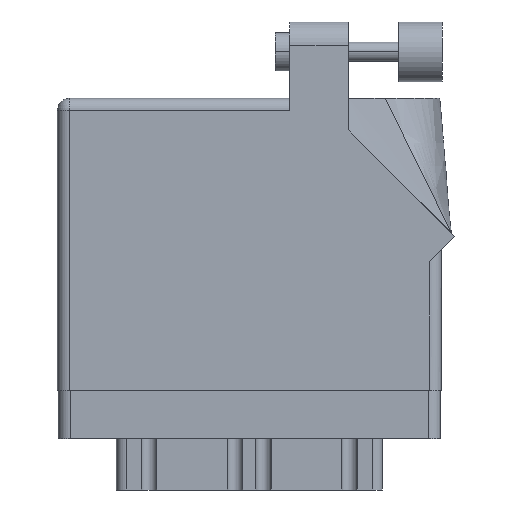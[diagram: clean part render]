
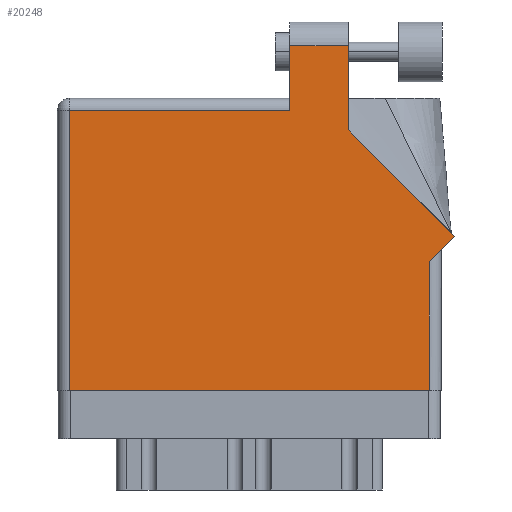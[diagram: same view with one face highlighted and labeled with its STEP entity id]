
A CAD part, front view. The second image highlights one B-rep face of the part: STEP entity #20248.
In plain terms, the highlighted face is planar.
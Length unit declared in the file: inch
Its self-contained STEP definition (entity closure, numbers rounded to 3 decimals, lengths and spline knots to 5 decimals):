
#191 = CARTESIAN_POINT ( 'NONE',  ( 1.948, 0., 0. ) ) ;
#868 = CARTESIAN_POINT ( 'NONE',  ( 2.08071, 0.80771, 0. ) ) ;
#1690 = CARTESIAN_POINT ( 'NONE',  ( 0., 1.53, 0. ) ) ;
#2049 = DIRECTION ( 'NONE',  ( 0., -1., 0. ) ) ;
#2469 = VECTOR ( 'NONE', #13653, 39.37008 ) ;
#2564 = EDGE_CURVE ( 'NONE', #34526, #6730, #16351, .T. ) ;
#2568 = CARTESIAN_POINT ( 'NONE',  ( 1.948, 0.737, 0. ) ) ;
#2931 = CARTESIAN_POINT ( 'NONE',  ( 1.524, 1.36442, 0. ) ) ;
#4004 = LINE ( 'NONE', #868, #5457 ) ;
#4192 = VECTOR ( 'NONE', #5695, 39.37008 ) ;
#4237 = DIRECTION ( 'NONE',  ( 0., 0., -1. ) ) ;
#4546 = ORIENTED_EDGE ( 'NONE', *, *, #4769, .T. ) ;
#4769 = EDGE_CURVE ( 'NONE', #14271, #34526, #4004, .T. ) ;
#4991 = VECTOR ( 'NONE', #36808, 39.37008 ) ;
#5081 = ORIENTED_EDGE ( 'NONE', *, *, #16974, .T. ) ;
#5451 = DIRECTION ( 'NONE',  ( -1., 0., 0. ) ) ;
#5457 = VECTOR ( 'NONE', #15938, 39.37008 ) ;
#5651 = EDGE_CURVE ( 'NONE', #19628, #32296, #12867, .T. ) ;
#5695 = DIRECTION ( 'NONE',  ( 0., 1., 0. ) ) ;
#6150 = EDGE_CURVE ( 'NONE', #12556, #30649, #23180, .T. ) ;
#6730 = VERTEX_POINT ( 'NONE', #27021 ) ;
#9202 = CARTESIAN_POINT ( 'NONE',  ( 2.01, 0.737, 0. ) ) ;
#9507 = DIRECTION ( 'NONE',  ( -1., 0., 0. ) ) ;
#10709 = EDGE_CURVE ( 'NONE', #12248, #14271, #27019, .T. ) ;
#11856 = AXIS2_PLACEMENT_3D ( 'NONE', #1690, #4237, #34006 ) ;
#12248 = VERTEX_POINT ( 'NONE', #29646 ) ;
#12556 = VERTEX_POINT ( 'NONE', #23153 ) ;
#12867 = LINE ( 'NONE', #22465, #2469 ) ;
#12920 = CARTESIAN_POINT ( 'NONE',  ( 0.062, 0., 0. ) ) ;
#12975 = ORIENTED_EDGE ( 'NONE', *, *, #19681, .T. ) ;
#13653 = DIRECTION ( 'NONE',  ( 0., -1., 0. ) ) ;
#13792 = CARTESIAN_POINT ( 'NONE',  ( 0.062, 0., 0. ) ) ;
#14181 = VECTOR ( 'NONE', #5451, 39.37008 ) ;
#14271 = VERTEX_POINT ( 'NONE', #23122 ) ;
#14471 = ORIENTED_EDGE ( 'NONE', *, *, #10709, .T. ) ;
#14861 = CARTESIAN_POINT ( 'NONE',  ( 1.217, 1.805, 0. ) ) ;
#15001 = LINE ( 'NONE', #33222, #16649 ) ;
#15307 = ORIENTED_EDGE ( 'NONE', *, *, #6150, .T. ) ;
#15938 = DIRECTION ( 'NONE',  ( -0.707, 0.707, 0. ) ) ;
#16351 = LINE ( 'NONE', #22430, #29589 ) ;
#16416 = EDGE_LOOP ( 'NONE', ( #38161, #33741, #23751, #5081, #15307, #12975, #36879, #14471, #4546 ) ) ;
#16649 = VECTOR ( 'NONE', #9507, 39.37008 ) ;
#16974 = EDGE_CURVE ( 'NONE', #32296, #12556, #15001, .T. ) ;
#18012 = DIRECTION ( 'NONE',  ( 0.707, 0.707, 0. ) ) ;
#19482 = DIRECTION ( 'NONE',  ( 0., 1., 0. ) ) ;
#19628 = VERTEX_POINT ( 'NONE', #14861 ) ;
#19681 = EDGE_CURVE ( 'NONE', #30649, #21785, #33084, .T. ) ;
#20248 = ADVANCED_FACE ( 'NONE', ( #30848 ), #31043, .F. ) ;
#21785 = VERTEX_POINT ( 'NONE', #191 ) ;
#22430 = CARTESIAN_POINT ( 'NONE',  ( 1.524, 1.36442, 0. ) ) ;
#22465 = CARTESIAN_POINT ( 'NONE',  ( 1.217, 1.53, 0. ) ) ;
#23122 = CARTESIAN_POINT ( 'NONE',  ( 2.08071, 0.80771, 0. ) ) ;
#23153 = CARTESIAN_POINT ( 'NONE',  ( 0.062, 1.468, 0. ) ) ;
#23180 = LINE ( 'NONE', #13792, #30400 ) ;
#23454 = LINE ( 'NONE', #38173, #14181 ) ;
#23470 = CARTESIAN_POINT ( 'NONE',  ( 1.217, 1.468, 0. ) ) ;
#23751 = ORIENTED_EDGE ( 'NONE', *, *, #5651, .T. ) ;
#25885 = VECTOR ( 'NONE', #18012, 39.37008 ) ;
#26836 = LINE ( 'NONE', #2568, #4192 ) ;
#27019 = LINE ( 'NONE', #9202, #25885 ) ;
#27021 = CARTESIAN_POINT ( 'NONE',  ( 1.524, 1.805, 0. ) ) ;
#27770 = CARTESIAN_POINT ( 'NONE',  ( 0., 0., 0. ) ) ;
#29589 = VECTOR ( 'NONE', #19482, 39.37008 ) ;
#29646 = CARTESIAN_POINT ( 'NONE',  ( 1.948, 0.675, 0. ) ) ;
#30400 = VECTOR ( 'NONE', #2049, 39.37008 ) ;
#30502 = EDGE_CURVE ( 'NONE', #21785, #12248, #26836, .T. ) ;
#30649 = VERTEX_POINT ( 'NONE', #12920 ) ;
#30848 = FACE_OUTER_BOUND ( 'NONE', #16416, .T. ) ;
#31043 = PLANE ( 'NONE',  #11856 ) ;
#32296 = VERTEX_POINT ( 'NONE', #23470 ) ;
#33084 = LINE ( 'NONE', #27770, #4991 ) ;
#33222 = CARTESIAN_POINT ( 'NONE',  ( 0., 1.468, 0. ) ) ;
#33741 = ORIENTED_EDGE ( 'NONE', *, *, #36496, .T. ) ;
#34006 = DIRECTION ( 'NONE',  ( -1., 0., 0. ) ) ;
#34526 = VERTEX_POINT ( 'NONE', #2931 ) ;
#36496 = EDGE_CURVE ( 'NONE', #6730, #19628, #23454, .T. ) ;
#36808 = DIRECTION ( 'NONE',  ( 1., 0., 0. ) ) ;
#36879 = ORIENTED_EDGE ( 'NONE', *, *, #30502, .T. ) ;
#38161 = ORIENTED_EDGE ( 'NONE', *, *, #2564, .T. ) ;
#38173 = CARTESIAN_POINT ( 'NONE',  ( 1.217, 1.805, 0. ) ) ;
